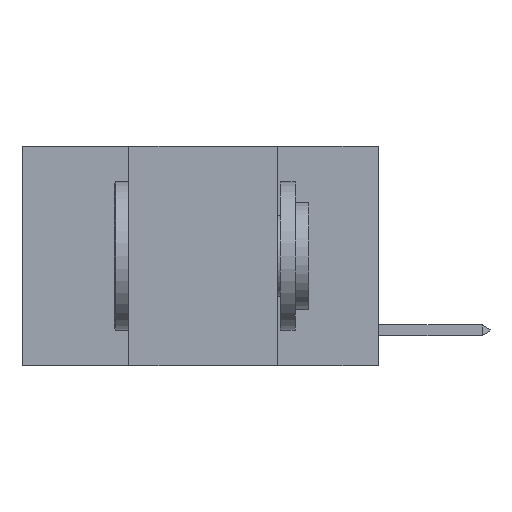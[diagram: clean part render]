
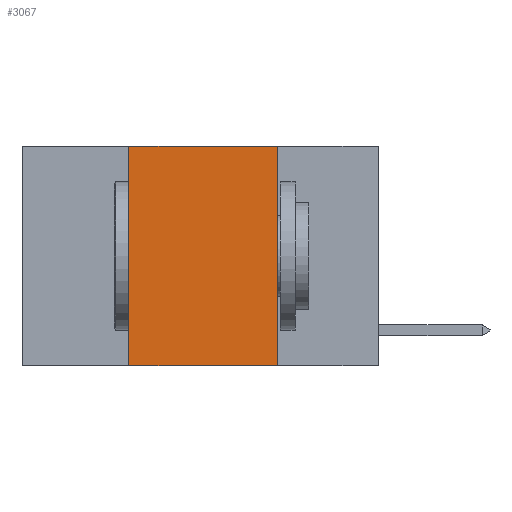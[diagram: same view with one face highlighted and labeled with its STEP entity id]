
A CAD part, left-side view. The second image highlights one B-rep face of the part: STEP entity #3067.
In plain terms, the highlighted planar face has unit normal (-1, 0, 0).
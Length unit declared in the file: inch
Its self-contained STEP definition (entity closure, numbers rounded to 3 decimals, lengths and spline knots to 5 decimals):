
#169 = VECTOR ( 'NONE', #11167, 39.37008 ) ;
#554 = ORIENTED_EDGE ( 'NONE', *, *, #9538, .F. ) ;
#986 = ORIENTED_EDGE ( 'NONE', *, *, #16374, .F. ) ;
#1418 = ORIENTED_EDGE ( 'NONE', *, *, #11091, .T. ) ;
#1672 = VERTEX_POINT ( 'NONE', #4378 ) ;
#1827 = CARTESIAN_POINT ( 'NONE',  ( 0., 0.17, 0. ) ) ;
#1869 = CARTESIAN_POINT ( 'NONE',  ( 0., 0.6, -0.37 ) ) ;
#3067 = ADVANCED_FACE ( 'NONE', ( #17225 ), #12439, .F. ) ;
#3414 = CARTESIAN_POINT ( 'NONE',  ( 0., 0.42, 0. ) ) ;
#4378 = CARTESIAN_POINT ( 'NONE',  ( 0., 0.17, -0.37 ) ) ;
#5159 = VECTOR ( 'NONE', #9871, 39.37008 ) ;
#7389 = ORIENTED_EDGE ( 'NONE', *, *, #10442, .F. ) ;
#7465 = LINE ( 'NONE', #11785, #14018 ) ;
#7597 = CARTESIAN_POINT ( 'NONE',  ( 0., 0.42, -0.37 ) ) ;
#7598 = CARTESIAN_POINT ( 'NONE',  ( 0., 0.17, 0. ) ) ;
#7884 = VERTEX_POINT ( 'NONE', #7597 ) ;
#9525 = EDGE_LOOP ( 'NONE', ( #7389, #554, #986, #1418 ) ) ;
#9538 = EDGE_CURVE ( 'NONE', #16784, #16439, #7465, .T. ) ;
#9871 = DIRECTION ( 'NONE',  ( 0., -1., 0. ) ) ;
#10442 = EDGE_CURVE ( 'NONE', #16439, #1672, #10870, .T. ) ;
#10449 = DIRECTION ( 'NONE',  ( 0., -1., 0. ) ) ;
#10870 = LINE ( 'NONE', #1827, #169 ) ;
#11091 = EDGE_CURVE ( 'NONE', #7884, #1672, #14400, .T. ) ;
#11167 = DIRECTION ( 'NONE',  ( 0., 0., -1. ) ) ;
#11785 = CARTESIAN_POINT ( 'NONE',  ( 0., 0.6, 0. ) ) ;
#12130 = DIRECTION ( 'NONE',  ( 0., 0., -1. ) ) ;
#12167 = DIRECTION ( 'NONE',  ( 1., 0., 0. ) ) ;
#12224 = CARTESIAN_POINT ( 'NONE',  ( 0., 0.6, 0. ) ) ;
#12424 = AXIS2_PLACEMENT_3D ( 'NONE', #12224, #12167, #12130 ) ;
#12439 = PLANE ( 'NONE',  #12424 ) ;
#12703 = DIRECTION ( 'NONE',  ( 0., 0., 1. ) ) ;
#13733 = LINE ( 'NONE', #3414, #14132 ) ;
#14018 = VECTOR ( 'NONE', #10449, 39.37008 ) ;
#14132 = VECTOR ( 'NONE', #12703, 39.37008 ) ;
#14400 = LINE ( 'NONE', #1869, #5159 ) ;
#16374 = EDGE_CURVE ( 'NONE', #7884, #16784, #13733, .T. ) ;
#16439 = VERTEX_POINT ( 'NONE', #7598 ) ;
#16784 = VERTEX_POINT ( 'NONE', #17076 ) ;
#17076 = CARTESIAN_POINT ( 'NONE',  ( 0., 0.42, 0. ) ) ;
#17225 = FACE_OUTER_BOUND ( 'NONE', #9525, .T. ) ;
